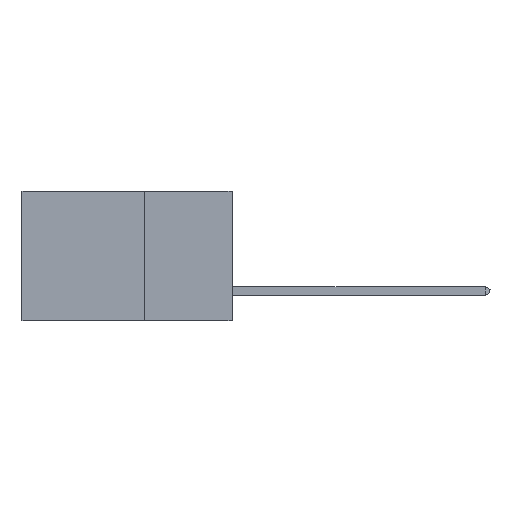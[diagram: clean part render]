
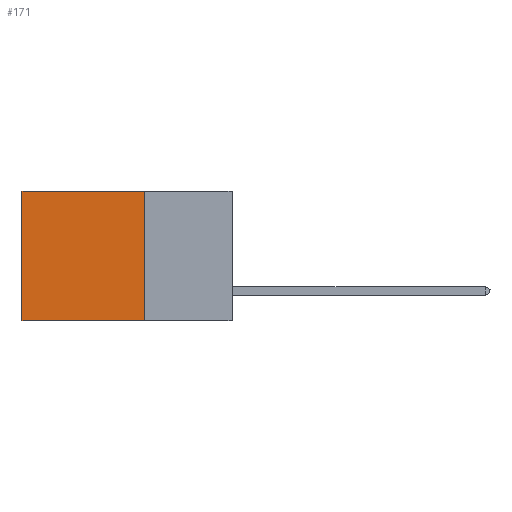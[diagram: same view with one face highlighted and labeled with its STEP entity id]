
A CAD part, left-side view. The second image highlights one B-rep face of the part: STEP entity #171.
In plain terms, the highlighted planar face has unit normal (-1, 0, 0).
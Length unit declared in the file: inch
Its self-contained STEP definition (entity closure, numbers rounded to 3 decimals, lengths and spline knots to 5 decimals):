
#171 = ADVANCED_FACE ( 'NONE', ( #15359 ), #4667, .F. ) ;
#245 = DIRECTION ( 'NONE',  ( 0., 0., -1. ) ) ;
#1756 = VERTEX_POINT ( 'NONE', #13852 ) ;
#1862 = LINE ( 'NONE', #5449, #8779 ) ;
#2135 = VECTOR ( 'NONE', #2978, 39.37008 ) ;
#2160 = ORIENTED_EDGE ( 'NONE', *, *, #15107, .F. ) ;
#2161 = EDGE_CURVE ( 'NONE', #3742, #1756, #3280, .T. ) ;
#2978 = DIRECTION ( 'NONE',  ( 0., 1., 0. ) ) ;
#3201 = CARTESIAN_POINT ( 'NONE',  ( 0.2875, 0.25, 0. ) ) ;
#3280 = LINE ( 'NONE', #17573, #2135 ) ;
#3288 = DIRECTION ( 'NONE',  ( 1., 0., 0. ) ) ;
#3289 = CARTESIAN_POINT ( 'NONE',  ( 0.2875, 0.25, 0. ) ) ;
#3742 = VERTEX_POINT ( 'NONE', #13705 ) ;
#3910 = VERTEX_POINT ( 'NONE', #14081 ) ;
#4518 = VECTOR ( 'NONE', #4912, 39.37008 ) ;
#4523 = EDGE_CURVE ( 'NONE', #3910, #1756, #1862, .T. ) ;
#4665 = VERTEX_POINT ( 'NONE', #11417 ) ;
#4667 = PLANE ( 'NONE',  #8431 ) ;
#4912 = DIRECTION ( 'NONE',  ( 0., 0., -1. ) ) ;
#5449 = CARTESIAN_POINT ( 'NONE',  ( 0.2875, 0.6, 0. ) ) ;
#6139 = CARTESIAN_POINT ( 'NONE',  ( 0.2875, 0.25, 0. ) ) ;
#7732 = LINE ( 'NONE', #3201, #10006 ) ;
#8431 = AXIS2_PLACEMENT_3D ( 'NONE', #6139, #3288, #245 ) ;
#8779 = VECTOR ( 'NONE', #17065, 39.37008 ) ;
#10006 = VECTOR ( 'NONE', #11971, 39.37008 ) ;
#11417 = CARTESIAN_POINT ( 'NONE',  ( 0.2875, 0.25, 0. ) ) ;
#11769 = EDGE_LOOP ( 'NONE', ( #14955, #14368, #2160, #17624 ) ) ;
#11971 = DIRECTION ( 'NONE',  ( 0., 1., 0. ) ) ;
#12819 = LINE ( 'NONE', #3289, #4518 ) ;
#13705 = CARTESIAN_POINT ( 'NONE',  ( 0.2875, 0.25, -0.37 ) ) ;
#13852 = CARTESIAN_POINT ( 'NONE',  ( 0.2875, 0.6, -0.37 ) ) ;
#14081 = CARTESIAN_POINT ( 'NONE',  ( 0.2875, 0.6, 0. ) ) ;
#14368 = ORIENTED_EDGE ( 'NONE', *, *, #2161, .F. ) ;
#14955 = ORIENTED_EDGE ( 'NONE', *, *, #4523, .T. ) ;
#15107 = EDGE_CURVE ( 'NONE', #4665, #3742, #12819, .T. ) ;
#15359 = FACE_OUTER_BOUND ( 'NONE', #11769, .T. ) ;
#16272 = EDGE_CURVE ( 'NONE', #4665, #3910, #7732, .T. ) ;
#17065 = DIRECTION ( 'NONE',  ( 0., 0., -1. ) ) ;
#17573 = CARTESIAN_POINT ( 'NONE',  ( 0.2875, 0.25, -0.37 ) ) ;
#17624 = ORIENTED_EDGE ( 'NONE', *, *, #16272, .T. ) ;
